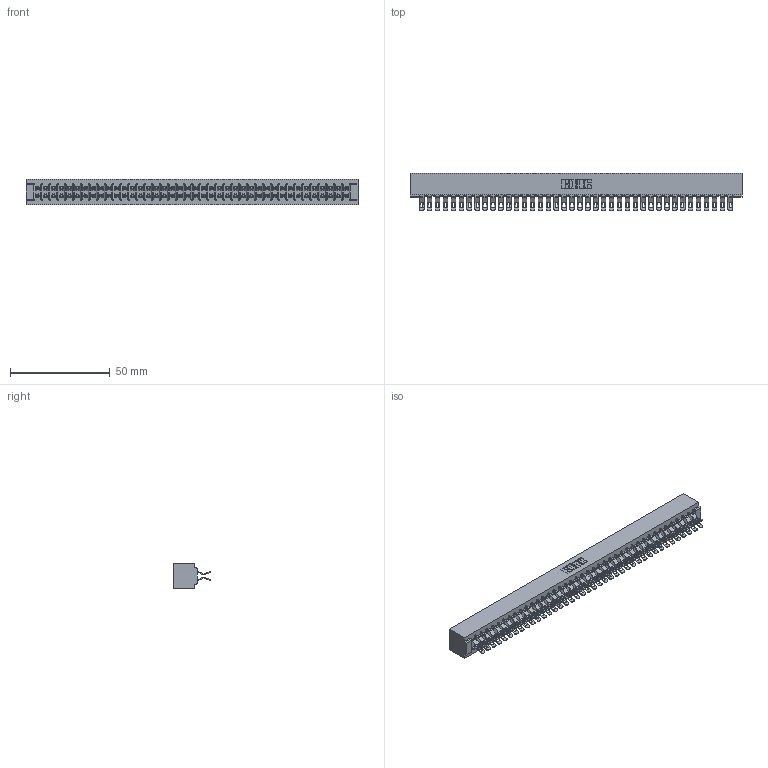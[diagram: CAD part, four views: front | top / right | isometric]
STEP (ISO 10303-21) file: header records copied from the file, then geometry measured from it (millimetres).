
FILE_DESCRIPTION (( 'STEP AP203' ), '1' );
FILE_NAME ('807-080-555-201.STEP', '2021-07-20T16:46:14', ( '' ), ( '' ), 'SwSTEP 2.0', 'SolidWorks 2020', '' );
FILE_SCHEMA (( 'CONFIG_CONTROL_DESIGN' ));
Length unit declared in the file: inch
Products named in the file (3): 807-080-555-201; 307-290-001_555; 807 Part_No Mounting Lugs
Assembly tree (81 placements, depth 2):
  807-080-555-201
    807 Part_No Mounting Lugs
    307-290-001_555  x80
Bounding box: 166.37 x 18.75 x 12.7 mm (x, y, z)
Volume: 18463.2 mm3; surface area: 24188.3 mm2
Topology: 81 solids, 81 shells, 5031 faces, 14779 edges, 9634 vertices
Faces by surface type: plane 2786, cylinder 2163, sphere 82
Entity records: 36077 total; most frequent: CARTESIAN_POINT 5904, ORIENTED_EDGE 5852, DIRECTION 5790, EDGE_CURVE 2926, VECTOR 2234, LINE 2234, VERTEX_POINT 1892, AXIS2_PLACEMENT_3D 1778
